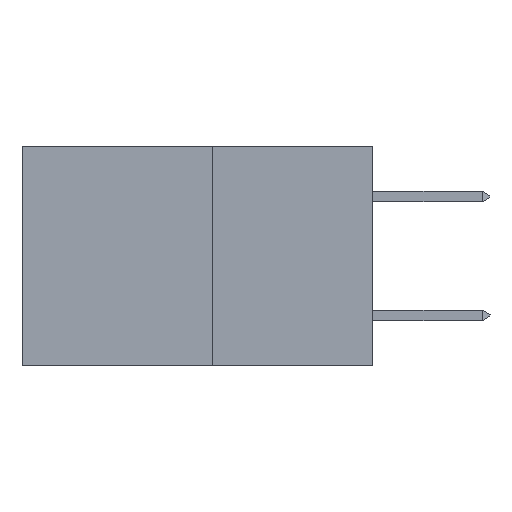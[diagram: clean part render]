
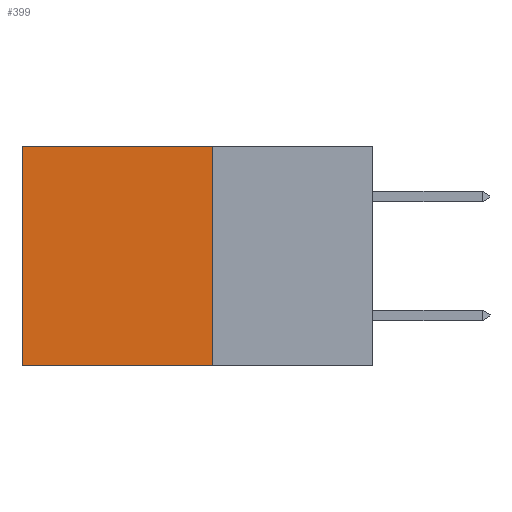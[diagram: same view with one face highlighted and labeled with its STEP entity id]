
A CAD part, left-side view. The second image highlights one B-rep face of the part: STEP entity #399.
In plain terms, the highlighted planar face has unit normal (-1, 0, 0).
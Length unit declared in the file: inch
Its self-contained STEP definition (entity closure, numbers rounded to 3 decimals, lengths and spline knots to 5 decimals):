
#399 = ADVANCED_FACE ( 'NONE', ( #12621 ), #10698, .F. ) ;
#2265 = EDGE_CURVE ( 'NONE', #15962, #7116, #2382, .T. ) ;
#2382 = LINE ( 'NONE', #15085, #21200 ) ;
#2819 = ORIENTED_EDGE ( 'NONE', *, *, #8624, .T. ) ;
#5291 = ORIENTED_EDGE ( 'NONE', *, *, #18268, .F. ) ;
#5321 = CARTESIAN_POINT ( 'NONE',  ( 0.277, 0.27, -0.37 ) ) ;
#5808 = ORIENTED_EDGE ( 'NONE', *, *, #21461, .F. ) ;
#5814 = DIRECTION ( 'NONE',  ( 0., 0., -1. ) ) ;
#7116 = VERTEX_POINT ( 'NONE', #16787 ) ;
#7357 = VECTOR ( 'NONE', #15856, 39.37008 ) ;
#8034 = CARTESIAN_POINT ( 'NONE',  ( 0.277, 0.59, 0. ) ) ;
#8624 = EDGE_CURVE ( 'NONE', #19893, #15962, #21402, .T. ) ;
#9923 = CARTESIAN_POINT ( 'NONE',  ( 0.277, 0.27, -0.37 ) ) ;
#10559 = AXIS2_PLACEMENT_3D ( 'NONE', #9923, #10751, #5814 ) ;
#10698 = PLANE ( 'NONE',  #10559 ) ;
#10751 = DIRECTION ( 'NONE',  ( 1., 0., 0. ) ) ;
#11208 = CARTESIAN_POINT ( 'NONE',  ( 0.277, 0.27, 0. ) ) ;
#12355 = DIRECTION ( 'NONE',  ( 0., 0., -1. ) ) ;
#12507 = VERTEX_POINT ( 'NONE', #16182 ) ;
#12621 = FACE_OUTER_BOUND ( 'NONE', #15642, .T. ) ;
#12674 = VECTOR ( 'NONE', #20104, 39.37008 ) ;
#13289 = CARTESIAN_POINT ( 'NONE',  ( 0.277, 0.27, 0. ) ) ;
#15085 = CARTESIAN_POINT ( 'NONE',  ( 0.277, 0.59, -0.37 ) ) ;
#15642 = EDGE_LOOP ( 'NONE', ( #17116, #5291, #5808, #2819 ) ) ;
#15856 = DIRECTION ( 'NONE',  ( 0., 1., 0. ) ) ;
#15962 = VERTEX_POINT ( 'NONE', #8034 ) ;
#16182 = CARTESIAN_POINT ( 'NONE',  ( 0.277, 0.27, -0.37 ) ) ;
#16567 = CARTESIAN_POINT ( 'NONE',  ( 0.277, 0.27, -0.37 ) ) ;
#16686 = VECTOR ( 'NONE', #21760, 39.37008 ) ;
#16787 = CARTESIAN_POINT ( 'NONE',  ( 0.277, 0.59, -0.37 ) ) ;
#17116 = ORIENTED_EDGE ( 'NONE', *, *, #2265, .T. ) ;
#17970 = LINE ( 'NONE', #16567, #12674 ) ;
#18268 = EDGE_CURVE ( 'NONE', #12507, #7116, #20873, .T. ) ;
#19893 = VERTEX_POINT ( 'NONE', #13289 ) ;
#20104 = DIRECTION ( 'NONE',  ( 0., 0., -1. ) ) ;
#20873 = LINE ( 'NONE', #5321, #7357 ) ;
#21200 = VECTOR ( 'NONE', #12355, 39.37008 ) ;
#21402 = LINE ( 'NONE', #11208, #16686 ) ;
#21461 = EDGE_CURVE ( 'NONE', #19893, #12507, #17970, .T. ) ;
#21760 = DIRECTION ( 'NONE',  ( 0., 1., 0. ) ) ;
